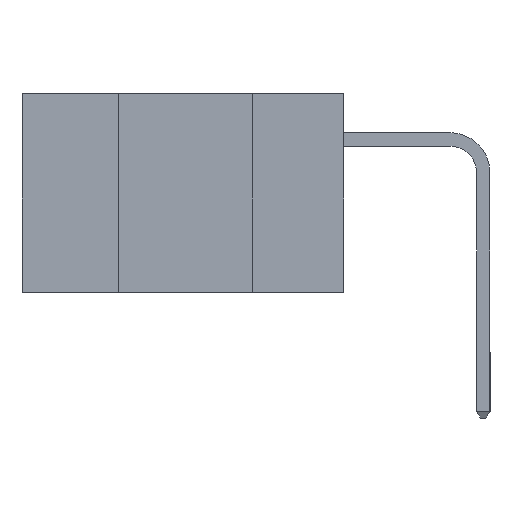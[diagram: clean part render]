
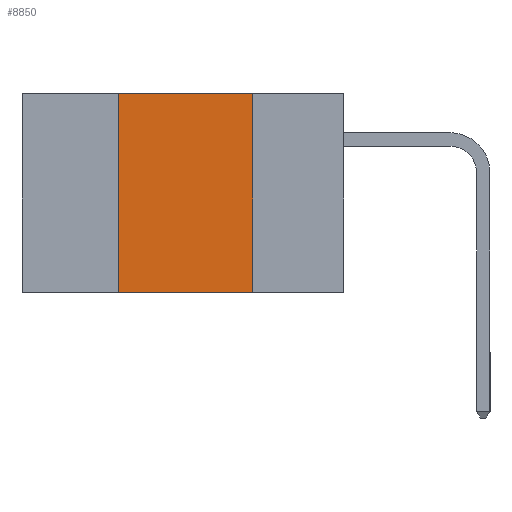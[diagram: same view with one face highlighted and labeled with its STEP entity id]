
A CAD part, left-side view. The second image highlights one B-rep face of the part: STEP entity #8850.
In plain terms, the highlighted planar face has unit normal (-1, 0, 0).
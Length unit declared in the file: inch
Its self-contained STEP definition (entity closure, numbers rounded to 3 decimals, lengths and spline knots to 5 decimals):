
#1483 = VECTOR ( 'NONE', #2293, 39.37008 ) ;
#2016 = VECTOR ( 'NONE', #10888, 39.37008 ) ;
#2293 = DIRECTION ( 'NONE',  ( 0., 0., -1. ) ) ;
#2546 = CARTESIAN_POINT ( 'NONE',  ( 0., 0.17, 0. ) ) ;
#2669 = CARTESIAN_POINT ( 'NONE',  ( 0., 0.42, 0. ) ) ;
#3430 = CARTESIAN_POINT ( 'NONE',  ( 0., 0.6, 0. ) ) ;
#3442 = ORIENTED_EDGE ( 'NONE', *, *, #17507, .F. ) ;
#3677 = EDGE_CURVE ( 'NONE', #23610, #6534, #7895, .T. ) ;
#3722 = CARTESIAN_POINT ( 'NONE',  ( 0., 0.42, 0. ) ) ;
#4222 = ORIENTED_EDGE ( 'NONE', *, *, #3677, .F. ) ;
#5620 = CARTESIAN_POINT ( 'NONE',  ( 0., 0.42, -0.37 ) ) ;
#6534 = VERTEX_POINT ( 'NONE', #31455 ) ;
#7010 = CARTESIAN_POINT ( 'NONE',  ( 0., 0.6, -0.37 ) ) ;
#7895 = LINE ( 'NONE', #2546, #1483 ) ;
#8850 = ADVANCED_FACE ( 'NONE', ( #17608 ), #25841, .F. ) ;
#10888 = DIRECTION ( 'NONE',  ( 0., 0., 1. ) ) ;
#10978 = LINE ( 'NONE', #7010, #16719 ) ;
#13580 = DIRECTION ( 'NONE',  ( 1., 0., 0. ) ) ;
#14000 = VERTEX_POINT ( 'NONE', #2669 ) ;
#16719 = VECTOR ( 'NONE', #24292, 39.37008 ) ;
#17507 = EDGE_CURVE ( 'NONE', #14000, #23610, #22103, .T. ) ;
#17608 = FACE_OUTER_BOUND ( 'NONE', #23255, .T. ) ;
#19085 = VERTEX_POINT ( 'NONE', #5620 ) ;
#21171 = AXIS2_PLACEMENT_3D ( 'NONE', #28208, #13580, #30580 ) ;
#21412 = ORIENTED_EDGE ( 'NONE', *, *, #24849, .F. ) ;
#22103 = LINE ( 'NONE', #3430, #27726 ) ;
#23255 = EDGE_LOOP ( 'NONE', ( #4222, #3442, #21412, #31315 ) ) ;
#23610 = VERTEX_POINT ( 'NONE', #26884 ) ;
#24292 = DIRECTION ( 'NONE',  ( 0., -1., 0. ) ) ;
#24467 = EDGE_CURVE ( 'NONE', #19085, #6534, #10978, .T. ) ;
#24849 = EDGE_CURVE ( 'NONE', #19085, #14000, #27156, .T. ) ;
#25841 = PLANE ( 'NONE',  #21171 ) ;
#26884 = CARTESIAN_POINT ( 'NONE',  ( 0., 0.17, 0. ) ) ;
#27156 = LINE ( 'NONE', #3722, #2016 ) ;
#27689 = DIRECTION ( 'NONE',  ( 0., -1., 0. ) ) ;
#27726 = VECTOR ( 'NONE', #27689, 39.37008 ) ;
#28208 = CARTESIAN_POINT ( 'NONE',  ( 0., 0.6, 0. ) ) ;
#30580 = DIRECTION ( 'NONE',  ( 0., 0., -1. ) ) ;
#31315 = ORIENTED_EDGE ( 'NONE', *, *, #24467, .T. ) ;
#31455 = CARTESIAN_POINT ( 'NONE',  ( 0., 0.17, -0.37 ) ) ;
